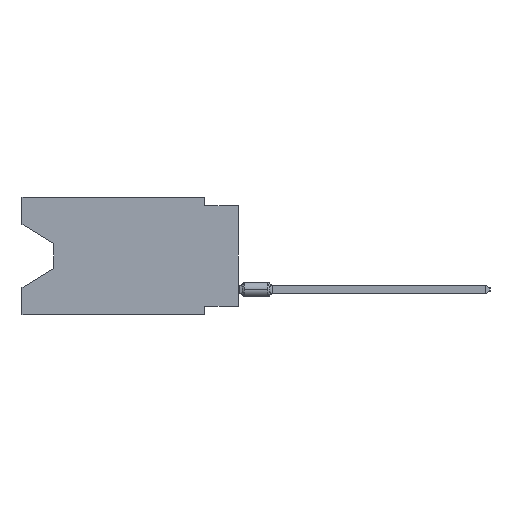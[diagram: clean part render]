
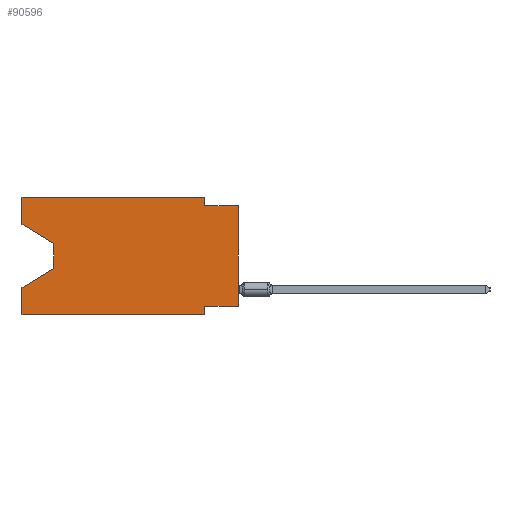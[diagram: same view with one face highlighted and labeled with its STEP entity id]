
A CAD part, left-side view. The second image highlights one B-rep face of the part: STEP entity #90596.
In plain terms, the highlighted planar face has unit normal (-1, 0, 0).
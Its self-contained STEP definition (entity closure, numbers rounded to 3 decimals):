
#154 = VECTOR ( 'NONE', #63256, 1000. ) ;
#611 = EDGE_CURVE ( 'NONE', #61807, #23633, #100066, .T. ) ;
#835 = LINE ( 'NONE', #89399, #56805 ) ;
#2506 = DIRECTION ( 'NONE',  ( 0., 0., -1. ) ) ;
#4000 = CARTESIAN_POINT ( 'NONE',  ( 0., 13.97, -3.505 ) ) ;
#6678 = EDGE_CURVE ( 'NONE', #23633, #95543, #74705, .T. ) ;
#9413 = CARTESIAN_POINT ( 'NONE',  ( 0., 16.383, -8.89 ) ) ;
#9968 = VERTEX_POINT ( 'NONE', #41869 ) ;
#11023 = CARTESIAN_POINT ( 'NONE',  ( 0., 16.383, -2.038 ) ) ;
#11929 = EDGE_CURVE ( 'NONE', #72214, #37719, #54874, .T. ) ;
#12786 = CARTESIAN_POINT ( 'NONE',  ( 0., 2.54, -8.89 ) ) ;
#13814 = PLANE ( 'NONE',  #99201 ) ;
#14681 = EDGE_CURVE ( 'NONE', #28115, #30339, #89430, .T. ) ;
#15814 = ORIENTED_EDGE ( 'NONE', *, *, #6678, .T. ) ;
#16434 = VECTOR ( 'NONE', #75864, 1000. ) ;
#17206 = DIRECTION ( 'NONE',  ( 0., 1., 0. ) ) ;
#18148 = VECTOR ( 'NONE', #17206, 1000. ) ;
#22209 = CARTESIAN_POINT ( 'NONE',  ( 0., 2.54, -8.255 ) ) ;
#22535 = ORIENTED_EDGE ( 'NONE', *, *, #99739, .T. ) ;
#23633 = VERTEX_POINT ( 'NONE', #4000 ) ;
#24590 = CARTESIAN_POINT ( 'NONE',  ( 0., 0., -8.255 ) ) ;
#25588 = CARTESIAN_POINT ( 'NONE',  ( 0., 0., -0.635 ) ) ;
#25816 = CARTESIAN_POINT ( 'NONE',  ( 0., 13.97, -5.385 ) ) ;
#27244 = CARTESIAN_POINT ( 'NONE',  ( 0., 13.97, -3.505 ) ) ;
#28115 = VERTEX_POINT ( 'NONE', #56098 ) ;
#29616 = CARTESIAN_POINT ( 'NONE',  ( 0., 16.383, 0. ) ) ;
#30339 = VERTEX_POINT ( 'NONE', #22209 ) ;
#30585 = CARTESIAN_POINT ( 'NONE',  ( 0., 16.383, 0. ) ) ;
#30856 = EDGE_CURVE ( 'NONE', #9968, #92844, #835, .T. ) ;
#30936 = EDGE_CURVE ( 'NONE', #92844, #39844, #97792, .T. ) ;
#34032 = DIRECTION ( 'NONE',  ( 0., 0., -1. ) ) ;
#35613 = VECTOR ( 'NONE', #92396, 1000. ) ;
#36390 = CARTESIAN_POINT ( 'NONE',  ( 0., 16.383, -2.038 ) ) ;
#37719 = VERTEX_POINT ( 'NONE', #74073 ) ;
#39844 = VERTEX_POINT ( 'NONE', #86417 ) ;
#41287 = EDGE_CURVE ( 'NONE', #95543, #37719, #58512, .T. ) ;
#41321 = VECTOR ( 'NONE', #58254, 1000. ) ;
#41622 = CARTESIAN_POINT ( 'NONE',  ( 0., 13.97, -5.385 ) ) ;
#41869 = CARTESIAN_POINT ( 'NONE',  ( 0., 2.54, 0. ) ) ;
#41898 = LINE ( 'NONE', #51373, #41321 ) ;
#42079 = CARTESIAN_POINT ( 'NONE',  ( 0., 2.54, -8.89 ) ) ;
#42100 = ORIENTED_EDGE ( 'NONE', *, *, #11929, .F. ) ;
#45099 = ORIENTED_EDGE ( 'NONE', *, *, #79450, .F. ) ;
#46220 = EDGE_CURVE ( 'NONE', #30339, #62029, #84482, .T. ) ;
#51373 = CARTESIAN_POINT ( 'NONE',  ( 0., 0., 0. ) ) ;
#53478 = EDGE_CURVE ( 'NONE', #28115, #39844, #41898, .T. ) ;
#53873 = FACE_OUTER_BOUND ( 'NONE', #60817, .T. ) ;
#54874 = LINE ( 'NONE', #93900, #65091 ) ;
#55362 = ORIENTED_EDGE ( 'NONE', *, *, #30936, .F. ) ;
#56098 = CARTESIAN_POINT ( 'NONE',  ( 0., 0., -8.255 ) ) ;
#56805 = VECTOR ( 'NONE', #34032, 1000. ) ;
#57393 = LINE ( 'NONE', #9413, #77833 ) ;
#57799 = ORIENTED_EDGE ( 'NONE', *, *, #53478, .T. ) ;
#58254 = DIRECTION ( 'NONE',  ( 0., 0., 1. ) ) ;
#58512 = LINE ( 'NONE', #25816, #77098 ) ;
#60817 = EDGE_LOOP ( 'NONE', ( #94722, #15814, #78024, #42100, #22535, #95684, #104053, #57799, #55362, #80210, #69061, #45099 ) ) ;
#61807 = VERTEX_POINT ( 'NONE', #36390 ) ;
#62029 = VERTEX_POINT ( 'NONE', #42079 ) ;
#62249 = CARTESIAN_POINT ( 'NONE',  ( 0., 16.383, -8.89 ) ) ;
#62304 = DIRECTION ( 'NONE',  ( 1., 0., 0. ) ) ;
#62790 = VECTOR ( 'NONE', #2506, 1000. ) ;
#63110 = CARTESIAN_POINT ( 'NONE',  ( 0., 2.54, -0.635 ) ) ;
#63256 = DIRECTION ( 'NONE',  ( 0., 0., 1. ) ) ;
#63823 = DIRECTION ( 'NONE',  ( 0., 0., 1. ) ) ;
#65091 = VECTOR ( 'NONE', #63823, 1000. ) ;
#65235 = EDGE_CURVE ( 'NONE', #77912, #9968, #94908, .T. ) ;
#69061 = ORIENTED_EDGE ( 'NONE', *, *, #65235, .F. ) ;
#69118 = CARTESIAN_POINT ( 'NONE',  ( 0., 16.383, 0. ) ) ;
#71646 = DIRECTION ( 'NONE',  ( 0., -1., 0. ) ) ;
#72214 = VERTEX_POINT ( 'NONE', #62249 ) ;
#74073 = CARTESIAN_POINT ( 'NONE',  ( 0., 16.383, -6.852 ) ) ;
#74705 = LINE ( 'NONE', #27244, #62790 ) ;
#75864 = DIRECTION ( 'NONE',  ( 0., -0.855, -0.519 ) ) ;
#77098 = VECTOR ( 'NONE', #80682, 1000. ) ;
#77602 = DIRECTION ( 'NONE',  ( 0., 0., -1. ) ) ;
#77833 = VECTOR ( 'NONE', #71646, 1000. ) ;
#77912 = VERTEX_POINT ( 'NONE', #80554 ) ;
#78024 = ORIENTED_EDGE ( 'NONE', *, *, #41287, .T. ) ;
#79450 = EDGE_CURVE ( 'NONE', #61807, #77912, #86996, .T. ) ;
#80120 = VECTOR ( 'NONE', #93883, 1000. ) ;
#80210 = ORIENTED_EDGE ( 'NONE', *, *, #30856, .F. ) ;
#80554 = CARTESIAN_POINT ( 'NONE',  ( 0., 16.383, 0. ) ) ;
#80682 = DIRECTION ( 'NONE',  ( 0., 0.855, -0.519 ) ) ;
#82517 = DIRECTION ( 'NONE',  ( 0., -1., 0. ) ) ;
#84482 = LINE ( 'NONE', #12786, #35613 ) ;
#86417 = CARTESIAN_POINT ( 'NONE',  ( 0., 0., -0.635 ) ) ;
#86996 = LINE ( 'NONE', #30585, #154 ) ;
#89399 = CARTESIAN_POINT ( 'NONE',  ( 0., 2.54, 0. ) ) ;
#89430 = LINE ( 'NONE', #24590, #18148 ) ;
#90596 = ADVANCED_FACE ( 'NONE', ( #53873 ), #13814, .F. ) ;
#92396 = DIRECTION ( 'NONE',  ( 0., 0., -1. ) ) ;
#92844 = VERTEX_POINT ( 'NONE', #63110 ) ;
#93883 = DIRECTION ( 'NONE',  ( 0., -1., 0. ) ) ;
#93892 = VECTOR ( 'NONE', #82517, 1000. ) ;
#93900 = CARTESIAN_POINT ( 'NONE',  ( 0., 16.383, 0. ) ) ;
#94722 = ORIENTED_EDGE ( 'NONE', *, *, #611, .T. ) ;
#94908 = LINE ( 'NONE', #69118, #80120 ) ;
#95543 = VERTEX_POINT ( 'NONE', #41622 ) ;
#95684 = ORIENTED_EDGE ( 'NONE', *, *, #46220, .F. ) ;
#97792 = LINE ( 'NONE', #25588, #93892 ) ;
#99201 = AXIS2_PLACEMENT_3D ( 'NONE', #29616, #62304, #77602 ) ;
#99739 = EDGE_CURVE ( 'NONE', #72214, #62029, #57393, .T. ) ;
#100066 = LINE ( 'NONE', #11023, #16434 ) ;
#104053 = ORIENTED_EDGE ( 'NONE', *, *, #14681, .F. ) ;
